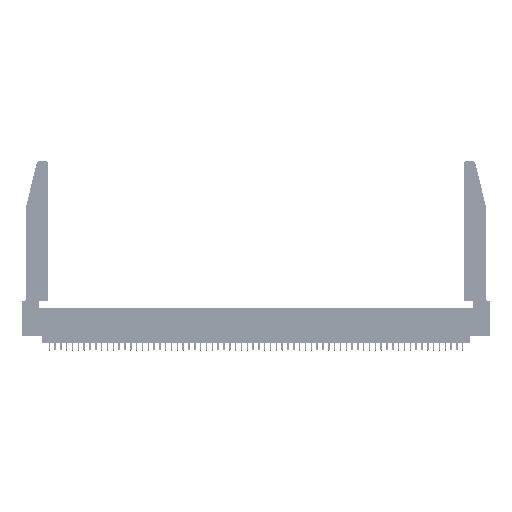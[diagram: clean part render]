
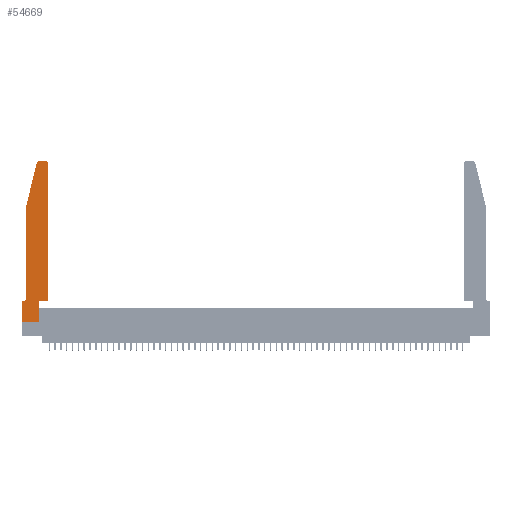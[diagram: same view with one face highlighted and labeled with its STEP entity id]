
A CAD part, top view. The second image highlights one B-rep face of the part: STEP entity #54669.
In plain terms, the highlighted planar face has unit normal (0, 0, 1).
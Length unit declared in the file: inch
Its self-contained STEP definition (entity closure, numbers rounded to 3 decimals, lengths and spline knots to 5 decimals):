
#978 = CARTESIAN_POINT ( 'NONE',  ( 0.2605, 2.75, 0.37 ) ) ;
#1098 = ORIENTED_EDGE ( 'NONE', *, *, #50186, .T. ) ;
#1308 = LINE ( 'NONE', #43510, #11759 ) ;
#2254 = DIRECTION ( 'NONE',  ( 1., 0., 0. ) ) ;
#3437 = CARTESIAN_POINT ( 'NONE',  ( 0.25487, 2.72718, 0.37 ) ) ;
#3667 = DIRECTION ( 'NONE',  ( 0., 1., 0. ) ) ;
#3838 = LINE ( 'NONE', #56777, #24780 ) ;
#3907 = VECTOR ( 'NONE', #55584, 39.37008 ) ;
#4414 = CARTESIAN_POINT ( 'NONE',  ( 0.4205, 2.75, 0.37 ) ) ;
#4433 = LINE ( 'NONE', #978, #14942 ) ;
#4528 = EDGE_CURVE ( 'NONE', #4696, #34182, #26216, .T. ) ;
#4696 = VERTEX_POINT ( 'NONE', #12631 ) ;
#5272 = VERTEX_POINT ( 'NONE', #38354 ) ;
#5280 = DIRECTION ( 'NONE',  ( 1., 0., 0. ) ) ;
#5672 = CARTESIAN_POINT ( 'NONE',  ( 0., 0.35, 0.37 ) ) ;
#6228 = CARTESIAN_POINT ( 'NONE',  ( 0., 0., 0.37 ) ) ;
#7163 = CARTESIAN_POINT ( 'NONE',  ( 0.0755, 0.35, 0.37 ) ) ;
#7237 = CARTESIAN_POINT ( 'NONE',  ( 0.284, 2.75, 0.37 ) ) ;
#7473 = EDGE_CURVE ( 'NONE', #11081, #16995, #31478, .T. ) ;
#7850 = DIRECTION ( 'NONE',  ( 0., 1., 0. ) ) ;
#8369 = CARTESIAN_POINT ( 'NONE',  ( 0.2865, 0.35, 0.37 ) ) ;
#9809 = LINE ( 'NONE', #22115, #32001 ) ;
#9910 = VECTOR ( 'NONE', #5280, 39.37008 ) ;
#9941 = DIRECTION ( 'NONE',  ( -1., 0., 0. ) ) ;
#10455 = CARTESIAN_POINT ( 'NONE',  ( 0.2865, 0., 0.37 ) ) ;
#10759 = VECTOR ( 'NONE', #2254, 39.37008 ) ;
#11081 = VERTEX_POINT ( 'NONE', #34758 ) ;
#11376 = PLANE ( 'NONE',  #27028 ) ;
#11759 = VECTOR ( 'NONE', #39065, 39.37008 ) ;
#12150 = CARTESIAN_POINT ( 'NONE',  ( 0.4505, 0.35, 0.37 ) ) ;
#12439 = EDGE_CURVE ( 'NONE', #5272, #38703, #1308, .T. ) ;
#12631 = CARTESIAN_POINT ( 'NONE',  ( 0.0055, 0.35, 0.37 ) ) ;
#12633 = CARTESIAN_POINT ( 'NONE',  ( 0.0755, 0.42, 0.37 ) ) ;
#12839 = EDGE_CURVE ( 'NONE', #34182, #36712, #14520, .T. ) ;
#13207 = VERTEX_POINT ( 'NONE', #4414 ) ;
#13681 = CIRCLE ( 'NONE', #55924, 0.03 ) ;
#14376 = ORIENTED_EDGE ( 'NONE', *, *, #7473, .T. ) ;
#14520 = LINE ( 'NONE', #6228, #24946 ) ;
#14616 = AXIS2_PLACEMENT_3D ( 'NONE', #52067, #25636, #56505 ) ;
#14942 = VECTOR ( 'NONE', #9941, 39.37008 ) ;
#15899 = CARTESIAN_POINT ( 'NONE',  ( 0., 0.35, 0.37 ) ) ;
#16382 = DIRECTION ( 'NONE',  ( 0., 0., -1. ) ) ;
#16995 = VERTEX_POINT ( 'NONE', #24833 ) ;
#17383 = ORIENTED_EDGE ( 'NONE', *, *, #34108, .T. ) ;
#18362 = ORIENTED_EDGE ( 'NONE', *, *, #51448, .T. ) ;
#18702 = VERTEX_POINT ( 'NONE', #10455 ) ;
#18864 = ORIENTED_EDGE ( 'NONE', *, *, #22197, .T. ) ;
#18934 = ORIENTED_EDGE ( 'NONE', *, *, #4528, .T. ) ;
#19800 = LINE ( 'NONE', #55335, #10759 ) ;
#19809 = VERTEX_POINT ( 'NONE', #3437 ) ;
#19951 = CIRCLE ( 'NONE', #14616, 0.03 ) ;
#20342 = DIRECTION ( 'NONE',  ( 0., 0., 1. ) ) ;
#21718 = LINE ( 'NONE', #49509, #9910 ) ;
#22115 = CARTESIAN_POINT ( 'NONE',  ( 0.0755, 2., 0.37 ) ) ;
#22197 = EDGE_CURVE ( 'NONE', #36712, #18702, #19800, .T. ) ;
#22663 = ORIENTED_EDGE ( 'NONE', *, *, #32879, .T. ) ;
#22993 = ORIENTED_EDGE ( 'NONE', *, *, #12439, .T. ) ;
#23616 = ORIENTED_EDGE ( 'NONE', *, *, #12839, .T. ) ;
#24447 = DIRECTION ( 'NONE',  ( 0., 0., 1. ) ) ;
#24780 = VECTOR ( 'NONE', #3667, 39.37008 ) ;
#24833 = CARTESIAN_POINT ( 'NONE',  ( 0.4505, 2.72, 0.37 ) ) ;
#24946 = VECTOR ( 'NONE', #50633, 39.37008 ) ;
#25636 = DIRECTION ( 'NONE',  ( 0., 0., 1. ) ) ;
#26216 = LINE ( 'NONE', #7163, #3907 ) ;
#26607 = DIRECTION ( 'NONE',  ( -0.239, -0.971, 0. ) ) ;
#27028 = AXIS2_PLACEMENT_3D ( 'NONE', #15899, #20342, #51272 ) ;
#27507 = ORIENTED_EDGE ( 'NONE', *, *, #30802, .T. ) ;
#30802 = EDGE_CURVE ( 'NONE', #38703, #4696, #56725, .T. ) ;
#31478 = LINE ( 'NONE', #12150, #53595 ) ;
#32001 = VECTOR ( 'NONE', #26607, 39.37008 ) ;
#32480 = VERTEX_POINT ( 'NONE', #7237 ) ;
#32879 = EDGE_CURVE ( 'NONE', #13207, #32480, #4433, .T. ) ;
#34108 = EDGE_CURVE ( 'NONE', #45794, #11081, #21718, .T. ) ;
#34182 = VERTEX_POINT ( 'NONE', #5672 ) ;
#34758 = CARTESIAN_POINT ( 'NONE',  ( 0.4505, 0.35, 0.37 ) ) ;
#36186 = EDGE_LOOP ( 'NONE', ( #22663, #40822, #44446, #22993, #27507, #18934, #23616, #18864, #18362, #17383, #14376, #1098 ) ) ;
#36712 = VERTEX_POINT ( 'NONE', #54742 ) ;
#38354 = CARTESIAN_POINT ( 'NONE',  ( 0.0755, 2., 0.37 ) ) ;
#38703 = VERTEX_POINT ( 'NONE', #12633 ) ;
#39065 = DIRECTION ( 'NONE',  ( 0., -1., 0. ) ) ;
#40822 = ORIENTED_EDGE ( 'NONE', *, *, #56954, .T. ) ;
#42866 = CARTESIAN_POINT ( 'NONE',  ( 0.0055, 0.42, 0.37 ) ) ;
#43510 = CARTESIAN_POINT ( 'NONE',  ( 0.0755, 2., 0.37 ) ) ;
#44446 = ORIENTED_EDGE ( 'NONE', *, *, #44528, .T. ) ;
#44528 = EDGE_CURVE ( 'NONE', #19809, #5272, #9809, .T. ) ;
#45794 = VERTEX_POINT ( 'NONE', #8369 ) ;
#47322 = DIRECTION ( 'NONE',  ( -1., 0., 0. ) ) ;
#49509 = CARTESIAN_POINT ( 'NONE',  ( 0.4505, 0.35, 0.37 ) ) ;
#50186 = EDGE_CURVE ( 'NONE', #16995, #13207, #19951, .T. ) ;
#50633 = DIRECTION ( 'NONE',  ( 0., -1., 0. ) ) ;
#50913 = CARTESIAN_POINT ( 'NONE',  ( 0.284, 2.72, 0.37 ) ) ;
#51272 = DIRECTION ( 'NONE',  ( 1., 0., 0. ) ) ;
#51448 = EDGE_CURVE ( 'NONE', #18702, #45794, #3838, .T. ) ;
#52044 = FACE_OUTER_BOUND ( 'NONE', #36186, .T. ) ;
#52067 = CARTESIAN_POINT ( 'NONE',  ( 0.4205, 2.72, 0.37 ) ) ;
#53595 = VECTOR ( 'NONE', #7850, 39.37008 ) ;
#53652 = AXIS2_PLACEMENT_3D ( 'NONE', #42866, #16382, #47322 ) ;
#54669 = ADVANCED_FACE ( 'NONE', ( #52044 ), #11376, .T. ) ;
#54742 = CARTESIAN_POINT ( 'NONE',  ( 0., 0., 0.37 ) ) ;
#55335 = CARTESIAN_POINT ( 'NONE',  ( 0., 0., 0.37 ) ) ;
#55338 = DIRECTION ( 'NONE',  ( 1., 0., 0. ) ) ;
#55584 = DIRECTION ( 'NONE',  ( -1., 0., 0. ) ) ;
#55924 = AXIS2_PLACEMENT_3D ( 'NONE', #50913, #24447, #55338 ) ;
#56505 = DIRECTION ( 'NONE',  ( 1., 0., 0. ) ) ;
#56725 = CIRCLE ( 'NONE', #53652, 0.07 ) ;
#56777 = CARTESIAN_POINT ( 'NONE',  ( 0.2865, 0.35, 0.37 ) ) ;
#56954 = EDGE_CURVE ( 'NONE', #32480, #19809, #13681, .T. ) ;
